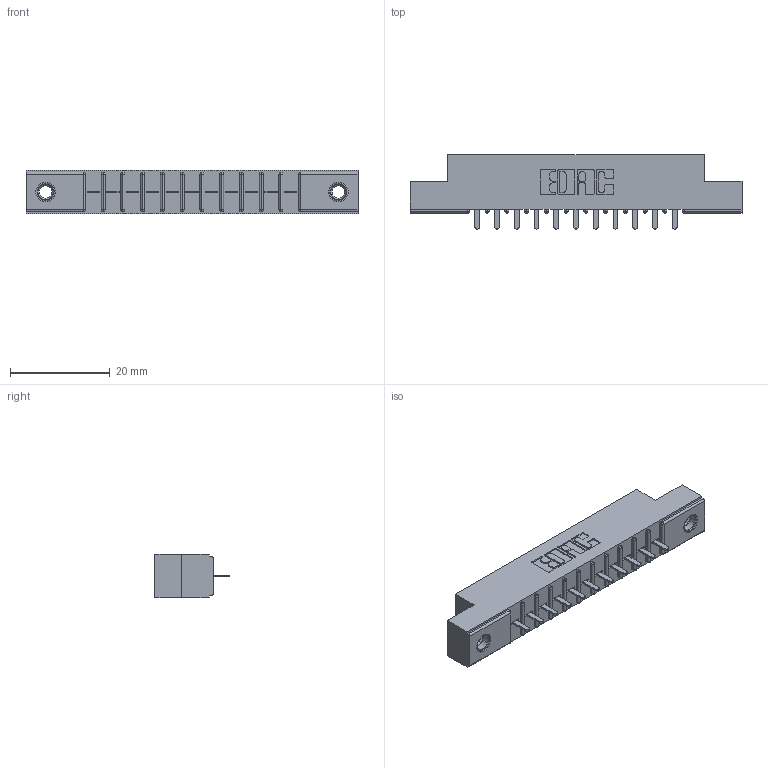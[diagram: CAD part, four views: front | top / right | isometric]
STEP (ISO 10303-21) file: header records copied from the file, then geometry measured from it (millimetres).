
FILE_DESCRIPTION (( 'STEP AP203' ), '1' );
FILE_NAME ('316-011-421-107.STEP', '2020-09-22T15:50:58', ( '' ), ( '' ), 'SwSTEP 2.0', 'SolidWorks 2020', '' );
FILE_SCHEMA (( 'CONFIG_CONTROL_DESIGN' ));
Length unit declared in the file: inch
Products named in the file (4): 306-290-001_121; 306 Part_.156 Dia; 316-011-421-107; 345-250-001_345-250-005-103
Assembly tree (14 placements, depth 2):
  316-011-421-107
    306 Part_.156 Dia
    306-290-001_121  x11
    345-250-001_345-250-005-103  x2
Bounding box: 66.6 x 14.88 x 8.71 mm (x, y, z)
Volume: 4482.6 mm3; surface area: 6234.5 mm2
Topology: 14 solids, 14 shells, 946 faces, 2619 edges, 1678 vertices
Faces by surface type: plane 617, cylinder 269, sphere 44, cone 12, torus 4
Entity records: 15415 total; most frequent: CARTESIAN_POINT 2563, DIRECTION 2539, ORIENTED_EDGE 2530, EDGE_CURVE 1265, LINE 971, VECTOR 971, VERTEX_POINT 808, AXIS2_PLACEMENT_3D 784
